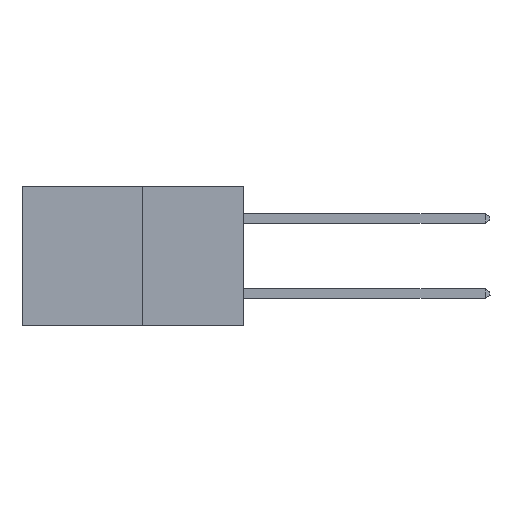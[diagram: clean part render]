
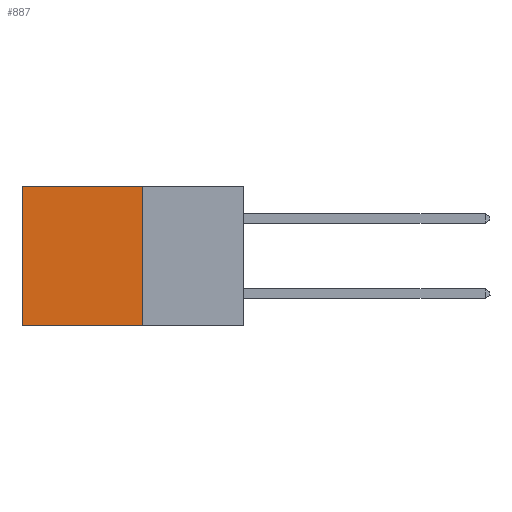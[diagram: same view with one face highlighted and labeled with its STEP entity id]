
A CAD part, left-side view. The second image highlights one B-rep face of the part: STEP entity #887.
In plain terms, the highlighted planar face has unit normal (-1, 0, 0).
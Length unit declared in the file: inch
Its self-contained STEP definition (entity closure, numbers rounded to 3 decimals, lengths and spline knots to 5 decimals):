
#619 = LINE ( 'NONE', #15748, #10975 ) ;
#887 = ADVANCED_FACE ( 'NONE', ( #17192 ), #12634, .F. ) ;
#1071 = LINE ( 'NONE', #22474, #6575 ) ;
#2514 = EDGE_LOOP ( 'NONE', ( #14219, #23921, #17671, #26342 ) ) ;
#2751 = CARTESIAN_POINT ( 'NONE',  ( 0.277, 0.27, 0. ) ) ;
#4473 = DIRECTION ( 'NONE',  ( 0., 1., 0. ) ) ;
#5511 = LINE ( 'NONE', #23908, #15774 ) ;
#5519 = DIRECTION ( 'NONE',  ( 0., 1., 0. ) ) ;
#6352 = VERTEX_POINT ( 'NONE', #14899 ) ;
#6575 = VECTOR ( 'NONE', #24531, 39.37008 ) ;
#8024 = EDGE_CURVE ( 'NONE', #6352, #23395, #619, .T. ) ;
#10975 = VECTOR ( 'NONE', #5519, 39.37008 ) ;
#12041 = VERTEX_POINT ( 'NONE', #13574 ) ;
#12251 = EDGE_CURVE ( 'NONE', #12041, #23395, #1071, .T. ) ;
#12634 = PLANE ( 'NONE',  #23258 ) ;
#13574 = CARTESIAN_POINT ( 'NONE',  ( 0.277, 0.59, 0. ) ) ;
#14219 = ORIENTED_EDGE ( 'NONE', *, *, #12251, .T. ) ;
#14899 = CARTESIAN_POINT ( 'NONE',  ( 0.277, 0.27, -0.37 ) ) ;
#15095 = EDGE_CURVE ( 'NONE', #18210, #6352, #5511, .T. ) ;
#15748 = CARTESIAN_POINT ( 'NONE',  ( 0.277, 0.27, -0.37 ) ) ;
#15774 = VECTOR ( 'NONE', #25931, 39.37008 ) ;
#17192 = FACE_OUTER_BOUND ( 'NONE', #2514, .T. ) ;
#17671 = ORIENTED_EDGE ( 'NONE', *, *, #15095, .F. ) ;
#18094 = VECTOR ( 'NONE', #4473, 39.37008 ) ;
#18210 = VERTEX_POINT ( 'NONE', #2751 ) ;
#18763 = DIRECTION ( 'NONE',  ( 1., 0., 0. ) ) ;
#18790 = DIRECTION ( 'NONE',  ( 0., 0., -1. ) ) ;
#21188 = CARTESIAN_POINT ( 'NONE',  ( 0.277, 0.27, -0.37 ) ) ;
#22474 = CARTESIAN_POINT ( 'NONE',  ( 0.277, 0.59, -0.37 ) ) ;
#23258 = AXIS2_PLACEMENT_3D ( 'NONE', #21188, #18763, #18790 ) ;
#23395 = VERTEX_POINT ( 'NONE', #26137 ) ;
#23571 = LINE ( 'NONE', #24893, #18094 ) ;
#23908 = CARTESIAN_POINT ( 'NONE',  ( 0.277, 0.27, -0.37 ) ) ;
#23921 = ORIENTED_EDGE ( 'NONE', *, *, #8024, .F. ) ;
#24531 = DIRECTION ( 'NONE',  ( 0., 0., -1. ) ) ;
#24893 = CARTESIAN_POINT ( 'NONE',  ( 0.277, 0.27, 0. ) ) ;
#25931 = DIRECTION ( 'NONE',  ( 0., 0., -1. ) ) ;
#26029 = EDGE_CURVE ( 'NONE', #18210, #12041, #23571, .T. ) ;
#26137 = CARTESIAN_POINT ( 'NONE',  ( 0.277, 0.59, -0.37 ) ) ;
#26342 = ORIENTED_EDGE ( 'NONE', *, *, #26029, .T. ) ;
